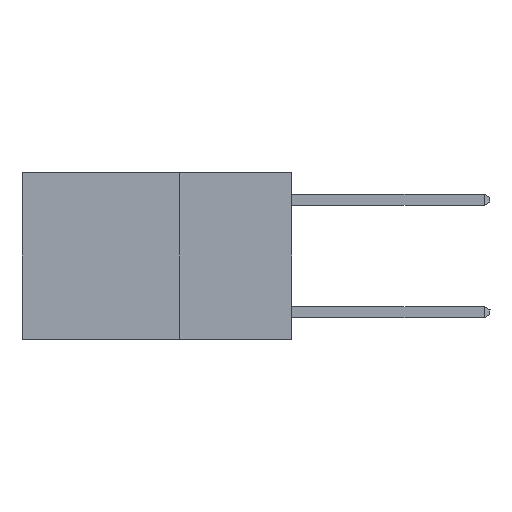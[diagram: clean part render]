
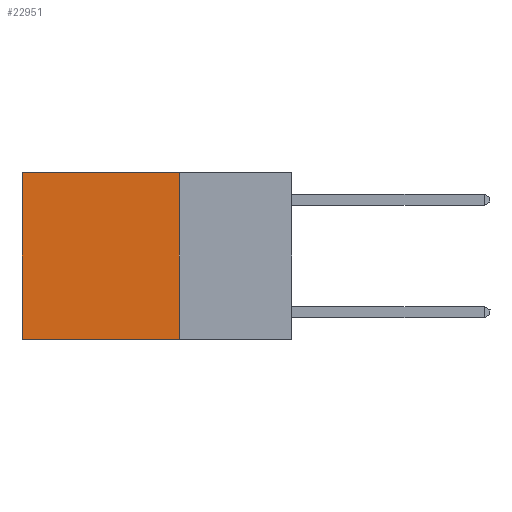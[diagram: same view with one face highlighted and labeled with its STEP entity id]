
A CAD part, left-side view. The second image highlights one B-rep face of the part: STEP entity #22951.
In plain terms, the highlighted planar face has unit normal (-1, 0, 0).
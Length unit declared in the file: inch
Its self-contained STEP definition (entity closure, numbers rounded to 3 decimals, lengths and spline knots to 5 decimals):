
#419 = VECTOR ( 'NONE', #30805, 39.37008 ) ;
#999 = ORIENTED_EDGE ( 'NONE', *, *, #25045, .T. ) ;
#1018 = ORIENTED_EDGE ( 'NONE', *, *, #22177, .T. ) ;
#1764 = VERTEX_POINT ( 'NONE', #2249 ) ;
#1801 = DIRECTION ( 'NONE',  ( 0., 1., 0. ) ) ;
#2249 = CARTESIAN_POINT ( 'NONE',  ( 0.2625, 0.25, -0.37 ) ) ;
#2513 = FACE_OUTER_BOUND ( 'NONE', #4435, .T. ) ;
#2797 = ORIENTED_EDGE ( 'NONE', *, *, #21127, .F. ) ;
#3085 = CARTESIAN_POINT ( 'NONE',  ( 0.2625, 0.25, 0. ) ) ;
#3103 = EDGE_CURVE ( 'NONE', #1764, #18520, #18943, .T. ) ;
#3121 = VERTEX_POINT ( 'NONE', #21374 ) ;
#4435 = EDGE_LOOP ( 'NONE', ( #1018, #8504, #2797, #999 ) ) ;
#4477 = VECTOR ( 'NONE', #27730, 39.37008 ) ;
#6387 = CARTESIAN_POINT ( 'NONE',  ( 0.2625, 0.25, 0. ) ) ;
#6454 = VERTEX_POINT ( 'NONE', #3085 ) ;
#7217 = LINE ( 'NONE', #30562, #19255 ) ;
#8504 = ORIENTED_EDGE ( 'NONE', *, *, #3103, .F. ) ;
#8543 = CARTESIAN_POINT ( 'NONE',  ( 0.2625, 0.6, 0. ) ) ;
#8801 = DIRECTION ( 'NONE',  ( 0., 0., -1. ) ) ;
#12076 = CARTESIAN_POINT ( 'NONE',  ( 0.2625, 0.25, 0. ) ) ;
#18520 = VERTEX_POINT ( 'NONE', #23746 ) ;
#18943 = LINE ( 'NONE', #28455, #419 ) ;
#19255 = VECTOR ( 'NONE', #1801, 39.37008 ) ;
#19918 = VECTOR ( 'NONE', #28724, 39.37008 ) ;
#20693 = LINE ( 'NONE', #12076, #19918 ) ;
#20809 = PLANE ( 'NONE',  #21438 ) ;
#21127 = EDGE_CURVE ( 'NONE', #6454, #1764, #20693, .T. ) ;
#21374 = CARTESIAN_POINT ( 'NONE',  ( 0.2625, 0.6, 0. ) ) ;
#21438 = AXIS2_PLACEMENT_3D ( 'NONE', #6387, #23223, #8801 ) ;
#22177 = EDGE_CURVE ( 'NONE', #3121, #18520, #23691, .T. ) ;
#22951 = ADVANCED_FACE ( 'NONE', ( #2513 ), #20809, .F. ) ;
#23223 = DIRECTION ( 'NONE',  ( 1., 0., 0. ) ) ;
#23691 = LINE ( 'NONE', #8543, #4477 ) ;
#23746 = CARTESIAN_POINT ( 'NONE',  ( 0.2625, 0.6, -0.37 ) ) ;
#25045 = EDGE_CURVE ( 'NONE', #6454, #3121, #7217, .T. ) ;
#27730 = DIRECTION ( 'NONE',  ( 0., 0., -1. ) ) ;
#28455 = CARTESIAN_POINT ( 'NONE',  ( 0.2625, 0.25, -0.37 ) ) ;
#28724 = DIRECTION ( 'NONE',  ( 0., 0., -1. ) ) ;
#30562 = CARTESIAN_POINT ( 'NONE',  ( 0.2625, 0.25, 0. ) ) ;
#30805 = DIRECTION ( 'NONE',  ( 0., 1., 0. ) ) ;
